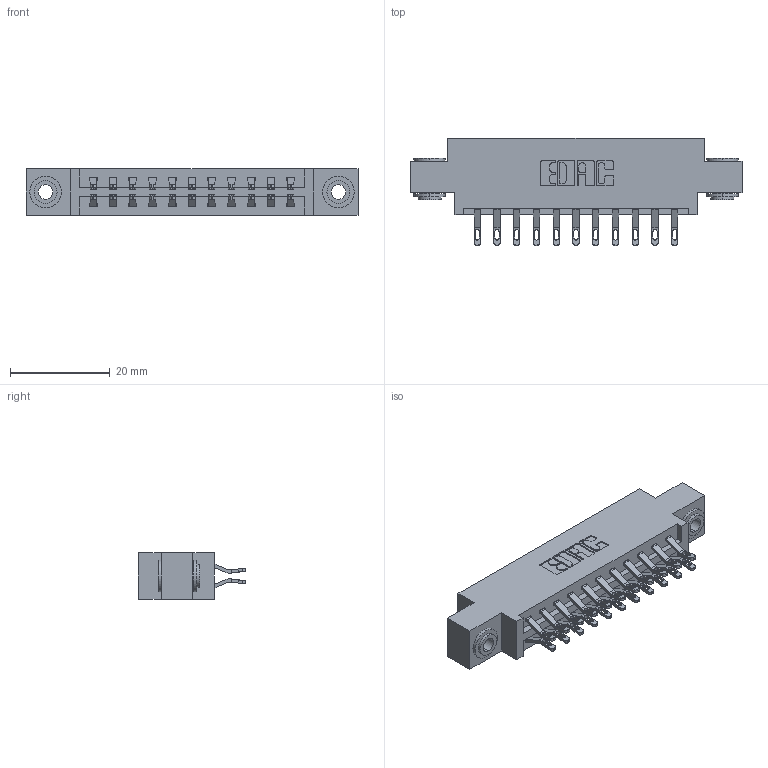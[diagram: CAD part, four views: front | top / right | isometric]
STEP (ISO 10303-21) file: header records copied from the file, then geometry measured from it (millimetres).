
FILE_DESCRIPTION (( 'STEP AP203' ), '1' );
FILE_NAME ('337-022-555-803.STEP', '2019-10-10T20:18:42', ( '' ), ( '' ), 'SwSTEP 2.0', 'SolidWorks 2016', '' );
FILE_SCHEMA (( 'CONFIG_CONTROL_DESIGN' ));
Length unit declared in the file: inch
Products named in the file (4): 337-022-555-803; 345-250-002_345-250-002-102; 337 Part_0.170 Offset - 0.156 Dia-TH; 345-292-001_555 Tail
Assembly tree (25 placements, depth 2):
  337-022-555-803
    337 Part_0.170 Offset - 0.156 Dia-TH
    345-292-001_555 Tail  x22
    345-250-002_345-250-002-102  x2
Bounding box: 66.6 x 21.47 x 9.4 mm (x, y, z)
Volume: 6571.8 mm3; surface area: 7701 mm2
Topology: 25 solids, 25 shells, 1476 faces, 4557 edges, 3034 vertices
Faces by surface type: plane 876, cylinder 592, cone 8
Entity records: 13646 total; most frequent: CARTESIAN_POINT 2335, ORIENTED_EDGE 2234, DIRECTION 2047, EDGE_CURVE 1117, VECTOR 945, LINE 945, VERTEX_POINT 742, AXIS2_PLACEMENT_3D 551
